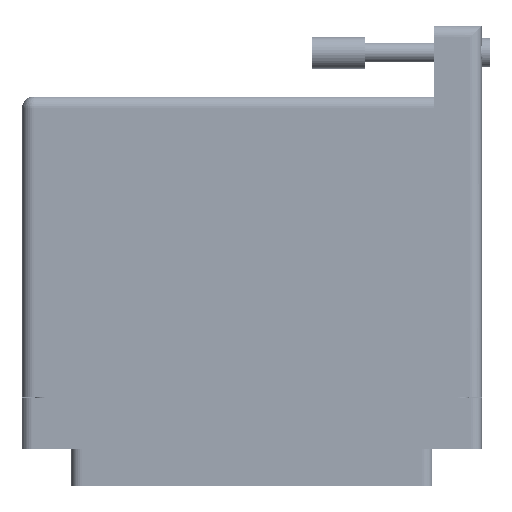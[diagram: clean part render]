
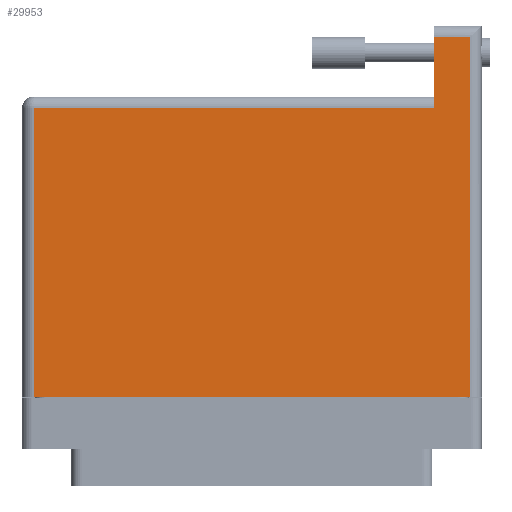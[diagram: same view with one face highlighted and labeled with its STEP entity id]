
A CAD part, front view. The second image highlights one B-rep face of the part: STEP entity #29953.
In plain terms, the highlighted face is planar.
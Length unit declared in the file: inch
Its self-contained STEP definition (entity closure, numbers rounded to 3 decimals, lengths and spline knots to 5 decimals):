
#285 = VERTEX_POINT ( 'NONE', #59855 ) ;
#2081 = DIRECTION ( 'NONE',  ( -1., 0., 0. ) ) ;
#2374 = PLANE ( 'NONE',  #15951 ) ;
#2810 = EDGE_CURVE ( 'NONE', #59956, #72556, #39560, .T. ) ;
#3252 = DIRECTION ( 'NONE',  ( -1., 0., 0. ) ) ;
#3567 = VECTOR ( 'NONE', #50133, 39.37008 ) ;
#4581 = CARTESIAN_POINT ( 'NONE',  ( 1.289, 2.025, 0.617 ) ) ;
#4701 = CARTESIAN_POINT ( 'NONE',  ( 1.079, 2.095, 0.617 ) ) ;
#5214 = VERTEX_POINT ( 'NONE', #72037 ) ;
#7137 = ORIENTED_EDGE ( 'NONE', *, *, #25874, .T. ) ;
#8534 = VERTEX_POINT ( 'NONE', #70293 ) ;
#9806 = EDGE_CURVE ( 'NONE', #285, #59956, #52138, .T. ) ;
#12309 = LINE ( 'NONE', #14720, #52235 ) ;
#14488 = DIRECTION ( 'NONE',  ( 0., 1., 0. ) ) ;
#14720 = CARTESIAN_POINT ( 'NONE',  ( -1.359, 2.025, 0.617 ) ) ;
#14843 = CARTESIAN_POINT ( 'NONE',  ( -1.289, -0.1, 0.617 ) ) ;
#15951 = AXIS2_PLACEMENT_3D ( 'NONE', #35895, #47252, #19543 ) ;
#19543 = DIRECTION ( 'NONE',  ( -1., 0., 0. ) ) ;
#20687 = EDGE_CURVE ( 'NONE', #72556, #8534, #12309, .T. ) ;
#20701 = EDGE_LOOP ( 'NONE', ( #22289, #7137, #40386, #63009, #44711, #42899 ) ) ;
#21985 = VECTOR ( 'NONE', #71286, 39.37008 ) ;
#22289 = ORIENTED_EDGE ( 'NONE', *, *, #36073, .T. ) ;
#23980 = VERTEX_POINT ( 'NONE', #44832 ) ;
#25491 = LINE ( 'NONE', #14843, #73559 ) ;
#25874 = EDGE_CURVE ( 'NONE', #5214, #285, #25491, .T. ) ;
#29953 = ADVANCED_FACE ( 'NONE', ( #45321 ), #2374, .F. ) ;
#35895 = CARTESIAN_POINT ( 'NONE',  ( -1.359, 1.675, 0.617 ) ) ;
#36073 = EDGE_CURVE ( 'NONE', #23980, #5214, #37377, .T. ) ;
#37355 = LINE ( 'NONE', #4701, #3567 ) ;
#37377 = LINE ( 'NONE', #54211, #52436 ) ;
#39560 = LINE ( 'NONE', #55166, #47524 ) ;
#40386 = ORIENTED_EDGE ( 'NONE', *, *, #9806, .T. ) ;
#42899 = ORIENTED_EDGE ( 'NONE', *, *, #61290, .T. ) ;
#44711 = ORIENTED_EDGE ( 'NONE', *, *, #20687, .T. ) ;
#44832 = CARTESIAN_POINT ( 'NONE',  ( 1.079, 1.605, 0.617 ) ) ;
#45321 = FACE_OUTER_BOUND ( 'NONE', #20701, .T. ) ;
#47252 = DIRECTION ( 'NONE',  ( 0., 0., -1. ) ) ;
#47524 = VECTOR ( 'NONE', #14488, 39.37008 ) ;
#50133 = DIRECTION ( 'NONE',  ( 0., -1., 0. ) ) ;
#52138 = LINE ( 'NONE', #70539, #21985 ) ;
#52235 = VECTOR ( 'NONE', #3252, 39.37008 ) ;
#52436 = VECTOR ( 'NONE', #2081, 39.37008 ) ;
#54211 = CARTESIAN_POINT ( 'NONE',  ( -1.359, 1.605, 0.617 ) ) ;
#55166 = CARTESIAN_POINT ( 'NONE',  ( 1.289, 2.095, 0.617 ) ) ;
#59855 = CARTESIAN_POINT ( 'NONE',  ( -1.289, -0.1, 0.617 ) ) ;
#59956 = VERTEX_POINT ( 'NONE', #60610 ) ;
#60209 = DIRECTION ( 'NONE',  ( 0., -1., 0. ) ) ;
#60610 = CARTESIAN_POINT ( 'NONE',  ( 1.289, -0.1, 0.617 ) ) ;
#61290 = EDGE_CURVE ( 'NONE', #8534, #23980, #37355, .T. ) ;
#63009 = ORIENTED_EDGE ( 'NONE', *, *, #2810, .T. ) ;
#70293 = CARTESIAN_POINT ( 'NONE',  ( 1.079, 2.025, 0.617 ) ) ;
#70539 = CARTESIAN_POINT ( 'NONE',  ( -1.359, -0.1, 0.617 ) ) ;
#71286 = DIRECTION ( 'NONE',  ( 1., 0., 0. ) ) ;
#72037 = CARTESIAN_POINT ( 'NONE',  ( -1.289, 1.605, 0.617 ) ) ;
#72556 = VERTEX_POINT ( 'NONE', #4581 ) ;
#73559 = VECTOR ( 'NONE', #60209, 39.37008 ) ;
